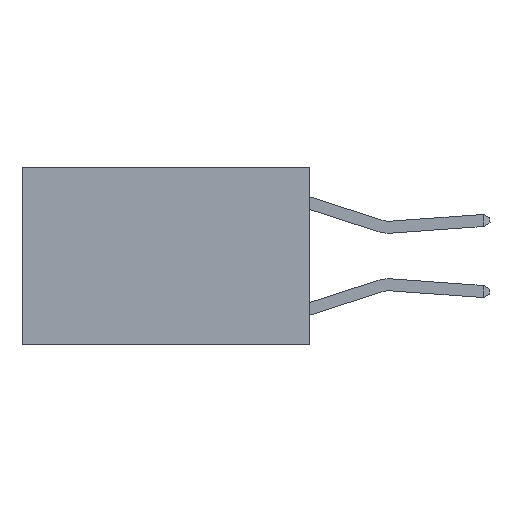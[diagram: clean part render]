
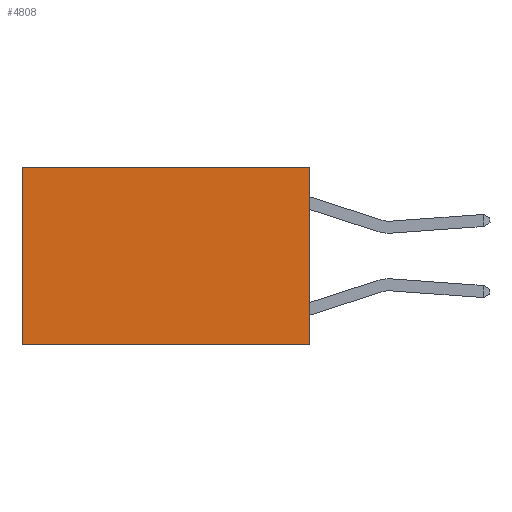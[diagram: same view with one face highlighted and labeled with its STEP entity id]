
A CAD part, left-side view. The second image highlights one B-rep face of the part: STEP entity #4808.
In plain terms, the highlighted planar face has unit normal (-1, 0, 0).
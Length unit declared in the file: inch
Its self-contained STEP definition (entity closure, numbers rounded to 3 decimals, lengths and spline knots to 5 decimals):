
#369 = DIRECTION ( 'NONE',  ( 0., 0., -1. ) ) ;
#694 = CARTESIAN_POINT ( 'NONE',  ( 0.2625, 0., 0. ) ) ;
#1120 = VERTEX_POINT ( 'NONE', #2531 ) ;
#1185 = LINE ( 'NONE', #4837, #5275 ) ;
#1795 = EDGE_CURVE ( 'NONE', #2289, #1120, #5150, .T. ) ;
#1898 = ORIENTED_EDGE ( 'NONE', *, *, #2632, .F. ) ;
#1927 = CARTESIAN_POINT ( 'NONE',  ( 0.2625, 0.6, 0. ) ) ;
#1941 = VECTOR ( 'NONE', #6977, 39.37008 ) ;
#2289 = VERTEX_POINT ( 'NONE', #8479 ) ;
#2360 = DIRECTION ( 'NONE',  ( 0., 0., -1. ) ) ;
#2531 = CARTESIAN_POINT ( 'NONE',  ( 0.2625, 0.6, -0.37 ) ) ;
#2632 = EDGE_CURVE ( 'NONE', #9242, #2920, #7723, .T. ) ;
#2920 = VERTEX_POINT ( 'NONE', #4686 ) ;
#3241 = DIRECTION ( 'NONE',  ( 0., 1., 0. ) ) ;
#3760 = CARTESIAN_POINT ( 'NONE',  ( 0.2625, 0., -0.37 ) ) ;
#4577 = FACE_OUTER_BOUND ( 'NONE', #10122, .T. ) ;
#4686 = CARTESIAN_POINT ( 'NONE',  ( 0.2625, 0., -0.37 ) ) ;
#4808 = ADVANCED_FACE ( 'NONE', ( #4577 ), #6375, .F. ) ;
#4837 = CARTESIAN_POINT ( 'NONE',  ( 0.2625, 0., 0. ) ) ;
#5150 = LINE ( 'NONE', #1927, #7019 ) ;
#5204 = CARTESIAN_POINT ( 'NONE',  ( 0.2625, 0., 0. ) ) ;
#5275 = VECTOR ( 'NONE', #3241, 39.37008 ) ;
#5333 = ORIENTED_EDGE ( 'NONE', *, *, #1795, .T. ) ;
#5613 = VECTOR ( 'NONE', #369, 39.37008 ) ;
#6227 = LINE ( 'NONE', #3760, #1941 ) ;
#6255 = ORIENTED_EDGE ( 'NONE', *, *, #9353, .F. ) ;
#6375 = PLANE ( 'NONE',  #7492 ) ;
#6742 = CARTESIAN_POINT ( 'NONE',  ( 0.2625, 0., 0. ) ) ;
#6977 = DIRECTION ( 'NONE',  ( 0., 1., 0. ) ) ;
#7019 = VECTOR ( 'NONE', #8505, 39.37008 ) ;
#7180 = DIRECTION ( 'NONE',  ( 1., 0., 0. ) ) ;
#7401 = EDGE_CURVE ( 'NONE', #9242, #2289, #1185, .T. ) ;
#7492 = AXIS2_PLACEMENT_3D ( 'NONE', #694, #7180, #2360 ) ;
#7723 = LINE ( 'NONE', #6742, #5613 ) ;
#8094 = ORIENTED_EDGE ( 'NONE', *, *, #7401, .T. ) ;
#8479 = CARTESIAN_POINT ( 'NONE',  ( 0.2625, 0.6, 0. ) ) ;
#8505 = DIRECTION ( 'NONE',  ( 0., 0., -1. ) ) ;
#9242 = VERTEX_POINT ( 'NONE', #5204 ) ;
#9353 = EDGE_CURVE ( 'NONE', #2920, #1120, #6227, .T. ) ;
#10122 = EDGE_LOOP ( 'NONE', ( #5333, #6255, #1898, #8094 ) ) ;
